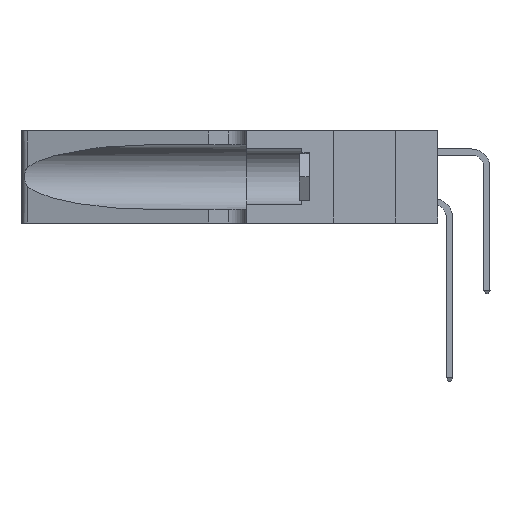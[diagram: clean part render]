
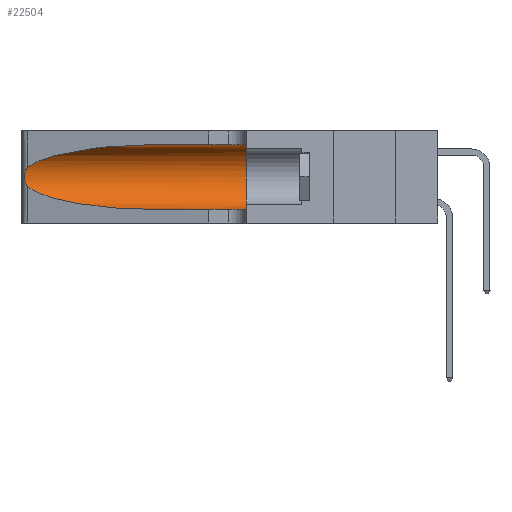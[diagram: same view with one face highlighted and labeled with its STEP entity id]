
A CAD part, left-side view. The second image highlights one B-rep face of the part: STEP entity #22504.
In plain terms, the highlighted cylindrical face has radius 3.308 mm (diameter 6.617 mm), a partial arc.
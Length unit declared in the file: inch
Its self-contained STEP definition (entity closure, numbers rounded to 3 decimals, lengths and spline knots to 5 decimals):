
#20 = CARTESIAN_POINT ( 'NONE',  ( 0.25639, 1.23184, 0.21858 ) ) ;
#3363 = LINE ( 'NONE', #40787, #19737 ) ;
#3411 = CARTESIAN_POINT ( 'NONE',  ( 0.25854, 1.2359, 0.20912 ) ) ;
#3829 = CARTESIAN_POINT ( 'NONE',  ( 0.25487, 1.22718, 0.14631 ) ) ;
#4029 = CARTESIAN_POINT ( 'NONE',  ( 0.1305, 0.72297, 0.31525 ) ) ;
#4918 = ORIENTED_EDGE ( 'NONE', *, *, #36834, .F. ) ;
#5388 = DIRECTION ( 'NONE',  ( 0., -1., 0. ) ) ;
#5470 = LINE ( 'NONE', #35660, #38907 ) ;
#5535 = CARTESIAN_POINT ( 'NONE',  ( 0.25487, 1.22718, 0.14631 ) ) ;
#6116 = VERTEX_POINT ( 'NONE', #6271 ) ;
#6271 = CARTESIAN_POINT ( 'NONE',  ( 0.1305, 0.72297, 0.31525 ) ) ;
#6707 = ORIENTED_EDGE ( 'NONE', *, *, #40174, .F. ) ;
#6768 = CARTESIAN_POINT ( 'NONE',  ( 0.26075, 1.23896, 0.19203 ) ) ;
#7183 = CARTESIAN_POINT ( 'NONE',  ( 0.1305, 0.72297, 0.05475 ) ) ;
#8298 = DIRECTION ( 'NONE',  ( 0., 1., 0. ) ) ;
#8605 = EDGE_LOOP ( 'NONE', ( #14429, #10969, #25940, #17736, #6707, #4918 ) ) ;
#9382 = CARTESIAN_POINT ( 'NONE',  ( 0.1305, 0.35, 0.05475 ) ) ;
#9543 = CARTESIAN_POINT ( 'NONE',  ( 0.25487, 1.22718, 0.22369 ) ) ;
#10080 = CARTESIAN_POINT ( 'NONE',  ( 0.26017, 1.23833, 0.17102 ) ) ;
#10969 = ORIENTED_EDGE ( 'NONE', *, *, #37769, .T. ) ;
#11242 =( BOUNDED_CURVE ( )  B_SPLINE_CURVE ( 3, ( #4029, #23577, #13987, #36508 ),
 .UNSPECIFIED., .F., .T. ) 
 B_SPLINE_CURVE_WITH_KNOTS ( ( 4, 4 ),
 ( 1.5708, 2.84003 ),
 .UNSPECIFIED. ) 
 CURVE ( )  GEOMETRIC_REPRESENTATION_ITEM ( )  RATIONAL_B_SPLINE_CURVE ( ( 1., 0.87, 0.87, 1. ) ) 
 REPRESENTATION_ITEM ( '' )  );
#13230 = CARTESIAN_POINT ( 'NONE',  ( 0.25487, 1.22718, 0.22369 ) ) ;
#13372 = CARTESIAN_POINT ( 'NONE',  ( 0.25789, 1.23486, 0.15765 ) ) ;
#13987 = CARTESIAN_POINT ( 'NONE',  ( 0.2373, 1.15595, 0.28018 ) ) ;
#14429 = ORIENTED_EDGE ( 'NONE', *, *, #28841, .T. ) ;
#16352 = CARTESIAN_POINT ( 'NONE',  ( 0.1305, 0.72297, 0.05475 ) ) ;
#16617 = CARTESIAN_POINT ( 'NONE',  ( 0.25555, 1.22993, 0.14849 ) ) ;
#17546 = VERTEX_POINT ( 'NONE', #9382 ) ;
#17736 = ORIENTED_EDGE ( 'NONE', *, *, #19500, .T. ) ;
#18936 = CIRCLE ( 'NONE', #41507, 0.13025 ) ;
#19500 = EDGE_CURVE ( 'NONE', #35717, #17546, #5470, .T. ) ;
#19544 = CYLINDRICAL_SURFACE ( 'NONE', #20586, 0.13025 ) ;
#19737 = VECTOR ( 'NONE', #5388, 39.37008 ) ;
#20586 = AXIS2_PLACEMENT_3D ( 'NONE', #37086, #40335, #21045 ) ;
#21045 = DIRECTION ( 'NONE',  ( 0., 0., -1. ) ) ;
#21472 = VERTEX_POINT ( 'NONE', #41543 ) ;
#22504 = ADVANCED_FACE ( 'NONE', ( #36683 ), #19544, .F. ) ;
#22975 = CARTESIAN_POINT ( 'NONE',  ( 0.25787, 1.23484, 0.2124 ) ) ;
#23379 = CARTESIAN_POINT ( 'NONE',  ( 0.2373, 1.15595, 0.08982 ) ) ;
#23577 = CARTESIAN_POINT ( 'NONE',  ( 0.18966, 0.96281, 0.31525 ) ) ;
#24421 = EDGE_CURVE ( 'NONE', #40317, #35717, #26290, .T. ) ;
#25940 = ORIENTED_EDGE ( 'NONE', *, *, #24421, .T. ) ;
#26254 = CARTESIAN_POINT ( 'NONE',  ( 0.26018, 1.23835, 0.19895 ) ) ;
#26290 =( BOUNDED_CURVE ( )  B_SPLINE_CURVE ( 3, ( #3829, #23379, #26659, #7183 ),
 .UNSPECIFIED., .F., .T. ) 
 B_SPLINE_CURVE_WITH_KNOTS ( ( 4, 4 ),
 ( 3.44316, 4.71239 ),
 .UNSPECIFIED. ) 
 CURVE ( )  GEOMETRIC_REPRESENTATION_ITEM ( )  RATIONAL_B_SPLINE_CURVE ( ( 1., 0.87, 0.87, 1. ) ) 
 REPRESENTATION_ITEM ( '' )  );
#26659 = CARTESIAN_POINT ( 'NONE',  ( 0.18966, 0.96281, 0.05475 ) ) ;
#27722 = CARTESIAN_POINT ( 'NONE',  ( 0.1305, 0.35, 0.185 ) ) ;
#28841 = EDGE_CURVE ( 'NONE', #6116, #29536, #11242, .T. ) ;
#29439 = CARTESIAN_POINT ( 'NONE',  ( 0.26075, 1.23896, 0.178 ) ) ;
#29536 = VERTEX_POINT ( 'NONE', #9543 ) ;
#30634 = B_SPLINE_CURVE_WITH_KNOTS ( 'NONE', 3,
 ( #13230, #32531, #20, #22975, #3411, #26254, #6768, #29439, #10080, #32671, #13372, #35905, #16617, #39159 ),
 .UNSPECIFIED., .F., .F.,
 ( 4, 2, 2, 2, 2, 2, 4 ),
 ( 0., 0.00027, 0.00053, 0.00107, 0.0016, 0.00187, 0.00214 ),
 .UNSPECIFIED. ) ;
#30930 = DIRECTION ( 'NONE',  ( 0., 0., 1. ) ) ;
#32531 = CARTESIAN_POINT ( 'NONE',  ( 0.25555, 1.22994, 0.2215 ) ) ;
#32554 = DIRECTION ( 'NONE',  ( 0., -1., 0. ) ) ;
#32671 = CARTESIAN_POINT ( 'NONE',  ( 0.25856, 1.23593, 0.16098 ) ) ;
#35660 = CARTESIAN_POINT ( 'NONE',  ( 0.1305, 1.61858, 0.05475 ) ) ;
#35717 = VERTEX_POINT ( 'NONE', #16352 ) ;
#35905 = CARTESIAN_POINT ( 'NONE',  ( 0.25639, 1.23186, 0.15144 ) ) ;
#36508 = CARTESIAN_POINT ( 'NONE',  ( 0.25487, 1.22718, 0.22369 ) ) ;
#36683 = FACE_OUTER_BOUND ( 'NONE', #8605, .T. ) ;
#36834 = EDGE_CURVE ( 'NONE', #6116, #21472, #3363, .T. ) ;
#37086 = CARTESIAN_POINT ( 'NONE',  ( 0.1305, 1.61858, 0.185 ) ) ;
#37769 = EDGE_CURVE ( 'NONE', #29536, #40317, #30634, .T. ) ;
#38907 = VECTOR ( 'NONE', #32554, 39.37008 ) ;
#39159 = CARTESIAN_POINT ( 'NONE',  ( 0.25487, 1.22718, 0.14631 ) ) ;
#40174 = EDGE_CURVE ( 'NONE', #21472, #17546, #18936, .T. ) ;
#40317 = VERTEX_POINT ( 'NONE', #5535 ) ;
#40335 = DIRECTION ( 'NONE',  ( 0., -1., 0. ) ) ;
#40787 = CARTESIAN_POINT ( 'NONE',  ( 0.1305, 1.61858, 0.31525 ) ) ;
#41507 = AXIS2_PLACEMENT_3D ( 'NONE', #27722, #8298, #30930 ) ;
#41543 = CARTESIAN_POINT ( 'NONE',  ( 0.1305, 0.35, 0.31525 ) ) ;
